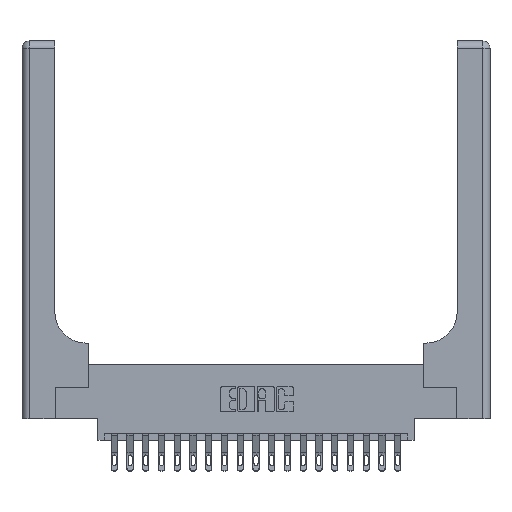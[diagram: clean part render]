
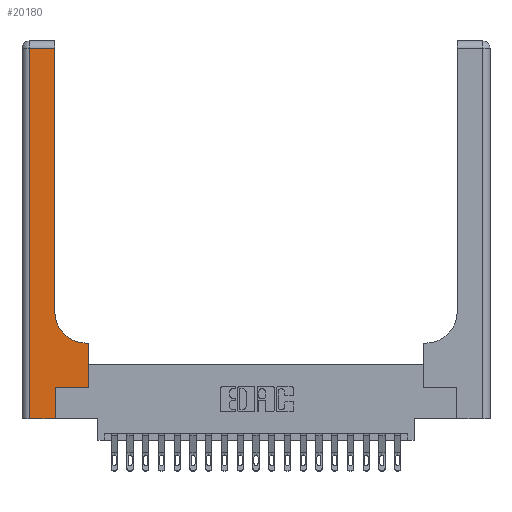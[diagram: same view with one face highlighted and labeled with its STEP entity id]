
A CAD part, top view. The second image highlights one B-rep face of the part: STEP entity #20180.
In plain terms, the highlighted planar face has unit normal (0, 0, 1).
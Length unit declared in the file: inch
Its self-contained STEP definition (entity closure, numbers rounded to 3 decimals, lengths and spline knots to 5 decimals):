
#1128 = ORIENTED_EDGE ( 'NONE', *, *, #7844, .T. ) ;
#1160 = VECTOR ( 'NONE', #7819, 39.37008 ) ;
#1324 = CARTESIAN_POINT ( 'NONE',  ( 0.265, 0., 0.37 ) ) ;
#1721 = VECTOR ( 'NONE', #7951, 39.37008 ) ;
#1910 = CARTESIAN_POINT ( 'NONE',  ( 0.06, 2.94, 0.37 ) ) ;
#2336 = CARTESIAN_POINT ( 'NONE',  ( 0.51, 0.6, 0.37 ) ) ;
#2355 = EDGE_CURVE ( 'NONE', #10615, #3449, #9423, .T. ) ;
#2682 = CARTESIAN_POINT ( 'NONE',  ( 0., 0., 0.37 ) ) ;
#2808 = DIRECTION ( 'NONE',  ( -1., 0., 0. ) ) ;
#2891 = LINE ( 'NONE', #13246, #15389 ) ;
#2934 = ORIENTED_EDGE ( 'NONE', *, *, #2355, .T. ) ;
#3224 = LINE ( 'NONE', #11396, #15699 ) ;
#3234 = CIRCLE ( 'NONE', #19476, 0.25 ) ;
#3412 = EDGE_CURVE ( 'NONE', #13759, #10615, #3234, .T. ) ;
#3449 = VERTEX_POINT ( 'NONE', #18274 ) ;
#3551 = VERTEX_POINT ( 'NONE', #10422 ) ;
#3607 = CARTESIAN_POINT ( 'NONE',  ( 0.26, 0.6, 0.37 ) ) ;
#3734 = ORIENTED_EDGE ( 'NONE', *, *, #3412, .T. ) ;
#3781 = CARTESIAN_POINT ( 'NONE',  ( 0.528, 0.25, 0.37 ) ) ;
#4417 = EDGE_CURVE ( 'NONE', #16143, #18750, #6537, .T. ) ;
#4602 = VECTOR ( 'NONE', #10605, 39.37008 ) ;
#4903 = DIRECTION ( 'NONE',  ( 0., 0., -1. ) ) ;
#5210 = EDGE_CURVE ( 'NONE', #10562, #9160, #2891, .T. ) ;
#5255 = DIRECTION ( 'NONE',  ( -1., 0., 0. ) ) ;
#5372 = CARTESIAN_POINT ( 'NONE',  ( 0.265, 0.25, 0.37 ) ) ;
#5583 = LINE ( 'NONE', #12779, #1721 ) ;
#5854 = VERTEX_POINT ( 'NONE', #1910 ) ;
#6021 = ORIENTED_EDGE ( 'NONE', *, *, #11847, .T. ) ;
#6166 = CARTESIAN_POINT ( 'NONE',  ( 0.26, 3., 0.37 ) ) ;
#6537 = LINE ( 'NONE', #2682, #18984 ) ;
#7074 = ORIENTED_EDGE ( 'NONE', *, *, #5210, .T. ) ;
#7259 = CARTESIAN_POINT ( 'NONE',  ( 0.06, 0., 0.37 ) ) ;
#7819 = DIRECTION ( 'NONE',  ( 0., 1., 0. ) ) ;
#7844 = EDGE_CURVE ( 'NONE', #18750, #3551, #17061, .T. ) ;
#7951 = DIRECTION ( 'NONE',  ( 0., -1., 0. ) ) ;
#8508 = EDGE_LOOP ( 'NONE', ( #2934, #16475, #8873, #17477, #1128, #6021, #7074, #15695, #3734 ) ) ;
#8873 = ORIENTED_EDGE ( 'NONE', *, *, #18758, .T. ) ;
#9160 = VERTEX_POINT ( 'NONE', #18145 ) ;
#9423 = LINE ( 'NONE', #6166, #1160 ) ;
#10422 = CARTESIAN_POINT ( 'NONE',  ( 0.265, 0.25, 0.37 ) ) ;
#10562 = VERTEX_POINT ( 'NONE', #3781 ) ;
#10605 = DIRECTION ( 'NONE',  ( 0., 1., 0. ) ) ;
#10615 = VERTEX_POINT ( 'NONE', #12193 ) ;
#10883 = FACE_OUTER_BOUND ( 'NONE', #8508, .T. ) ;
#10973 = PLANE ( 'NONE',  #14680 ) ;
#11396 = CARTESIAN_POINT ( 'NONE',  ( 0., 2.94, 0.37 ) ) ;
#11509 = EDGE_CURVE ( 'NONE', #9160, #13759, #20612, .T. ) ;
#11847 = EDGE_CURVE ( 'NONE', #3551, #10562, #18803, .T. ) ;
#11980 = VECTOR ( 'NONE', #5255, 39.37008 ) ;
#12193 = CARTESIAN_POINT ( 'NONE',  ( 0.26, 0.85, 0.37 ) ) ;
#12586 = DIRECTION ( 'NONE',  ( 0., 0., -1. ) ) ;
#12779 = CARTESIAN_POINT ( 'NONE',  ( 0.06, 3., 0.37 ) ) ;
#12934 = EDGE_CURVE ( 'NONE', #3449, #5854, #3224, .T. ) ;
#13038 = DIRECTION ( 'NONE',  ( -1., 0., 0. ) ) ;
#13246 = CARTESIAN_POINT ( 'NONE',  ( 0.528, 0.25, 0.37 ) ) ;
#13759 = VERTEX_POINT ( 'NONE', #2336 ) ;
#14487 = VECTOR ( 'NONE', #18378, 39.37008 ) ;
#14640 = CARTESIAN_POINT ( 'NONE',  ( 0.51, 0.85, 0.37 ) ) ;
#14680 = AXIS2_PLACEMENT_3D ( 'NONE', #17414, #12586, #2808 ) ;
#14858 = DIRECTION ( 'NONE',  ( 0., 1., 0. ) ) ;
#15389 = VECTOR ( 'NONE', #14858, 39.37008 ) ;
#15695 = ORIENTED_EDGE ( 'NONE', *, *, #11509, .T. ) ;
#15699 = VECTOR ( 'NONE', #13038, 39.37008 ) ;
#16143 = VERTEX_POINT ( 'NONE', #7259 ) ;
#16285 = DIRECTION ( 'NONE',  ( 1., 0., 0. ) ) ;
#16475 = ORIENTED_EDGE ( 'NONE', *, *, #12934, .T. ) ;
#17061 = LINE ( 'NONE', #20301, #4602 ) ;
#17414 = CARTESIAN_POINT ( 'NONE',  ( 0., 3., 0.37 ) ) ;
#17477 = ORIENTED_EDGE ( 'NONE', *, *, #4417, .T. ) ;
#18145 = CARTESIAN_POINT ( 'NONE',  ( 0.528, 0.6, 0.37 ) ) ;
#18274 = CARTESIAN_POINT ( 'NONE',  ( 0.26, 2.94, 0.37 ) ) ;
#18378 = DIRECTION ( 'NONE',  ( 1., 0., 0. ) ) ;
#18750 = VERTEX_POINT ( 'NONE', #1324 ) ;
#18758 = EDGE_CURVE ( 'NONE', #5854, #16143, #5583, .T. ) ;
#18803 = LINE ( 'NONE', #5372, #14487 ) ;
#18984 = VECTOR ( 'NONE', #19006, 39.37008 ) ;
#19006 = DIRECTION ( 'NONE',  ( 1., 0., 0. ) ) ;
#19476 = AXIS2_PLACEMENT_3D ( 'NONE', #14640, #4903, #16285 ) ;
#20180 = ADVANCED_FACE ( 'NONE', ( #10883 ), #10973, .F. ) ;
#20301 = CARTESIAN_POINT ( 'NONE',  ( 0.265, 0., 0.37 ) ) ;
#20612 = LINE ( 'NONE', #3607, #11980 ) ;
